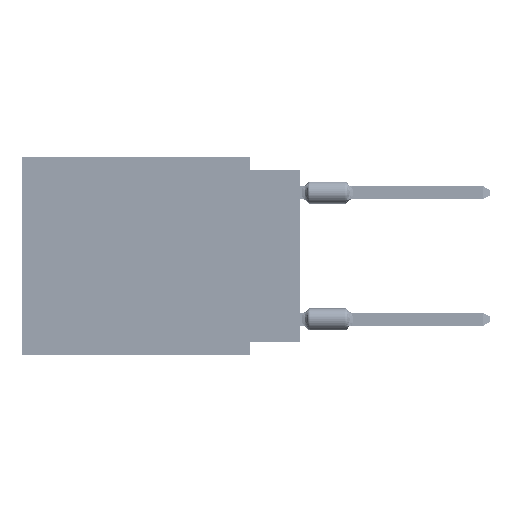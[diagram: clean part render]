
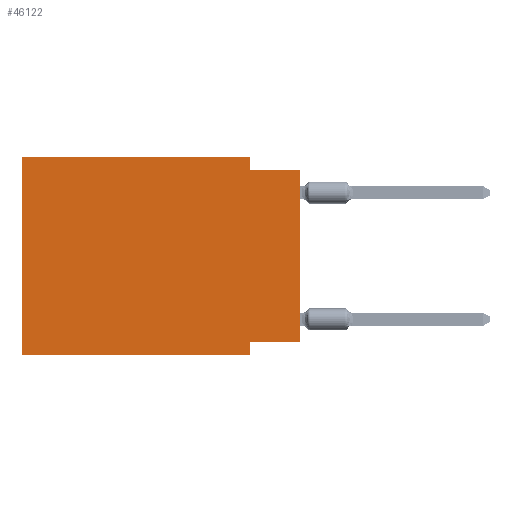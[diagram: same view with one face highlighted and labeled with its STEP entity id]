
A CAD part, left-side view. The second image highlights one B-rep face of the part: STEP entity #46122.
In plain terms, the highlighted planar face has unit normal (-1, 0, 0).
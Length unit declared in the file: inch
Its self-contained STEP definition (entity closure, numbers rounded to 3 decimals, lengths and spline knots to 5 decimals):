
#225 = CARTESIAN_POINT ( 'NONE',  ( 0., 0.1, -0.39 ) ) ;
#559 = LINE ( 'NONE', #63256, #10898 ) ;
#935 = DIRECTION ( 'NONE',  ( 0., -1., 0. ) ) ;
#4463 = CARTESIAN_POINT ( 'NONE',  ( 0., 0., -0.365 ) ) ;
#5323 = ORIENTED_EDGE ( 'NONE', *, *, #17968, .F. ) ;
#5847 = DIRECTION ( 'NONE',  ( 0., 0., -1. ) ) ;
#7349 = CARTESIAN_POINT ( 'NONE',  ( 0., 0., -0.025 ) ) ;
#7367 = EDGE_CURVE ( 'NONE', #19406, #47121, #49566, .T. ) ;
#7411 = DIRECTION ( 'NONE',  ( 1., 0., 0. ) ) ;
#7613 = CARTESIAN_POINT ( 'NONE',  ( 0., 0.1, -0.365 ) ) ;
#10898 = VECTOR ( 'NONE', #5847, 39.37008 ) ;
#11330 = EDGE_LOOP ( 'NONE', ( #33691, #64640, #5323, #73132, #56659, #39601, #52947, #16830 ) ) ;
#16830 = ORIENTED_EDGE ( 'NONE', *, *, #7367, .F. ) ;
#17241 = PLANE ( 'NONE',  #59274 ) ;
#17968 = EDGE_CURVE ( 'NONE', #32399, #53492, #34979, .T. ) ;
#17994 = DIRECTION ( 'NONE',  ( 0., 0., -1. ) ) ;
#19406 = VERTEX_POINT ( 'NONE', #4463 ) ;
#21222 = CARTESIAN_POINT ( 'NONE',  ( 0., 0., -0.365 ) ) ;
#21871 = EDGE_CURVE ( 'NONE', #59714, #49394, #68173, .T. ) ;
#22463 = DIRECTION ( 'NONE',  ( 0., -1., 0. ) ) ;
#22902 = FACE_OUTER_BOUND ( 'NONE', #11330, .T. ) ;
#23071 = CARTESIAN_POINT ( 'NONE',  ( 0., 0.1, -0.025 ) ) ;
#27660 = VECTOR ( 'NONE', #40453, 39.37008 ) ;
#30273 = LINE ( 'NONE', #48024, #40784 ) ;
#30607 = CARTESIAN_POINT ( 'NONE',  ( 0., 0., 0. ) ) ;
#32399 = VERTEX_POINT ( 'NONE', #70249 ) ;
#32903 = VERTEX_POINT ( 'NONE', #39360 ) ;
#33691 = ORIENTED_EDGE ( 'NONE', *, *, #54949, .T. ) ;
#34480 = EDGE_CURVE ( 'NONE', #59714, #32903, #30273, .T. ) ;
#34979 = LINE ( 'NONE', #52381, #38587 ) ;
#35163 = LINE ( 'NONE', #30607, #27660 ) ;
#38587 = VECTOR ( 'NONE', #17994, 39.37008 ) ;
#39360 = CARTESIAN_POINT ( 'NONE',  ( 0., 0.55, 0. ) ) ;
#39601 = ORIENTED_EDGE ( 'NONE', *, *, #21871, .T. ) ;
#40453 = DIRECTION ( 'NONE',  ( 0., 0., 1. ) ) ;
#40652 = VERTEX_POINT ( 'NONE', #53761 ) ;
#40784 = VECTOR ( 'NONE', #64645, 39.37008 ) ;
#42082 = LINE ( 'NONE', #7349, #48761 ) ;
#43546 = EDGE_CURVE ( 'NONE', #47121, #49394, #559, .T. ) ;
#44050 = LINE ( 'NONE', #45167, #69949 ) ;
#44263 = DIRECTION ( 'NONE',  ( 0., 1., 0. ) ) ;
#44637 = VECTOR ( 'NONE', #44263, 39.37008 ) ;
#45167 = CARTESIAN_POINT ( 'NONE',  ( 0., 0.55, 0. ) ) ;
#45955 = DIRECTION ( 'NONE',  ( 0., 0., -1. ) ) ;
#46122 = ADVANCED_FACE ( 'NONE', ( #22902 ), #17241, .F. ) ;
#47121 = VERTEX_POINT ( 'NONE', #7613 ) ;
#48024 = CARTESIAN_POINT ( 'NONE',  ( 0., 0.55, 0. ) ) ;
#48761 = VECTOR ( 'NONE', #935, 39.37008 ) ;
#49394 = VERTEX_POINT ( 'NONE', #225 ) ;
#49566 = LINE ( 'NONE', #21222, #44637 ) ;
#50795 = CARTESIAN_POINT ( 'NONE',  ( 0., 0.55, -0.39 ) ) ;
#52381 = CARTESIAN_POINT ( 'NONE',  ( 0., 0.1, 0. ) ) ;
#52947 = ORIENTED_EDGE ( 'NONE', *, *, #43546, .F. ) ;
#53492 = VERTEX_POINT ( 'NONE', #23071 ) ;
#53761 = CARTESIAN_POINT ( 'NONE',  ( 0., 0., -0.025 ) ) ;
#54503 = VECTOR ( 'NONE', #22463, 39.37008 ) ;
#54949 = EDGE_CURVE ( 'NONE', #19406, #40652, #35163, .T. ) ;
#56659 = ORIENTED_EDGE ( 'NONE', *, *, #34480, .F. ) ;
#57319 = EDGE_CURVE ( 'NONE', #32903, #32399, #44050, .T. ) ;
#59274 = AXIS2_PLACEMENT_3D ( 'NONE', #69357, #7411, #45955 ) ;
#59714 = VERTEX_POINT ( 'NONE', #67951 ) ;
#63256 = CARTESIAN_POINT ( 'NONE',  ( 0., 0.1, -0.39 ) ) ;
#64421 = EDGE_CURVE ( 'NONE', #53492, #40652, #42082, .T. ) ;
#64640 = ORIENTED_EDGE ( 'NONE', *, *, #64421, .F. ) ;
#64645 = DIRECTION ( 'NONE',  ( 0., 0., 1. ) ) ;
#67075 = DIRECTION ( 'NONE',  ( 0., -1., 0. ) ) ;
#67951 = CARTESIAN_POINT ( 'NONE',  ( 0., 0.55, -0.39 ) ) ;
#68173 = LINE ( 'NONE', #50795, #54503 ) ;
#69357 = CARTESIAN_POINT ( 'NONE',  ( 0., 0.55, 0. ) ) ;
#69949 = VECTOR ( 'NONE', #67075, 39.37008 ) ;
#70249 = CARTESIAN_POINT ( 'NONE',  ( 0., 0.1, 0. ) ) ;
#73132 = ORIENTED_EDGE ( 'NONE', *, *, #57319, .F. ) ;
